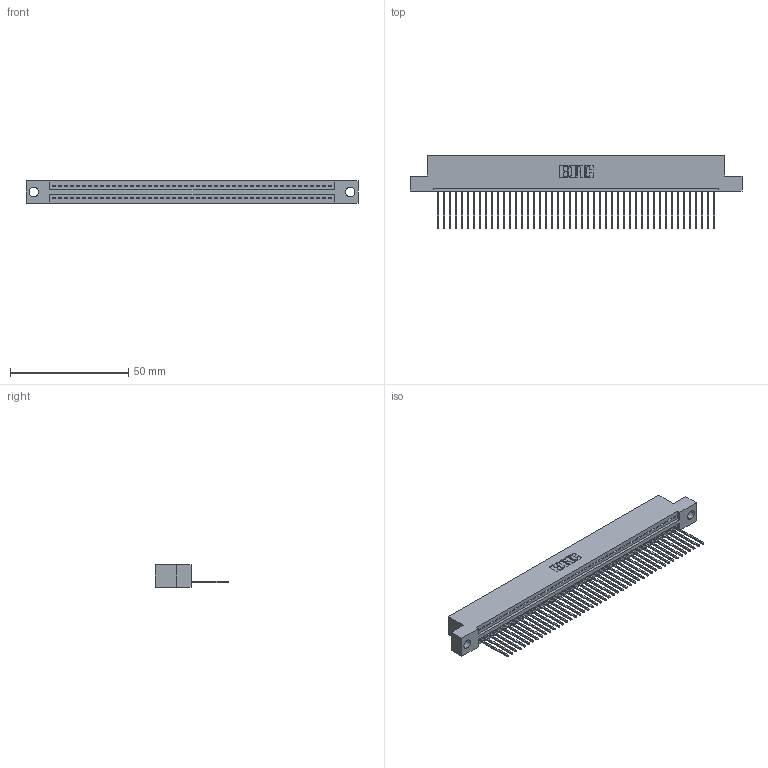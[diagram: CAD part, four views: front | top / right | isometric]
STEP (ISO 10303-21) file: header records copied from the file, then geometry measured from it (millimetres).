
FILE_DESCRIPTION (( 'STEP AP203' ), '1' );
FILE_NAME ('345-047-542-104.STEP', '2021-05-26T15:14:11', ( '' ), ( '' ), 'SwSTEP 2.0', 'SolidWorks 2020', '' );
FILE_SCHEMA (( 'CONFIG_CONTROL_DESIGN' ));
Length unit declared in the file: inch
Products named in the file (3): 345 Part_Flush Mounting Lugs - 0.156 Dia-TI; 345-047-542-104; 345-292-001_345-293-142
Assembly tree (48 placements, depth 2):
  345-047-542-104
    345 Part_Flush Mounting Lugs - 0.156 Dia-TI
    345-292-001_345-293-142  x47
Bounding box: 140.59 x 31.29 x 9.4 mm (x, y, z)
Volume: 13392.9 mm3; surface area: 18369.7 mm2
Topology: 48 solids, 48 shells, 2866 faces, 8649 edges, 5702 vertices
Faces by surface type: plane 1974, cylinder 892
Entity records: 35137 total; most frequent: CARTESIAN_POINT 6095, ORIENTED_EDGE 6074, DIRECTION 5315, EDGE_CURVE 3037, LINE 2717, VECTOR 2717, VERTEX_POINT 2022, AXIS2_PLACEMENT_3D 1299
